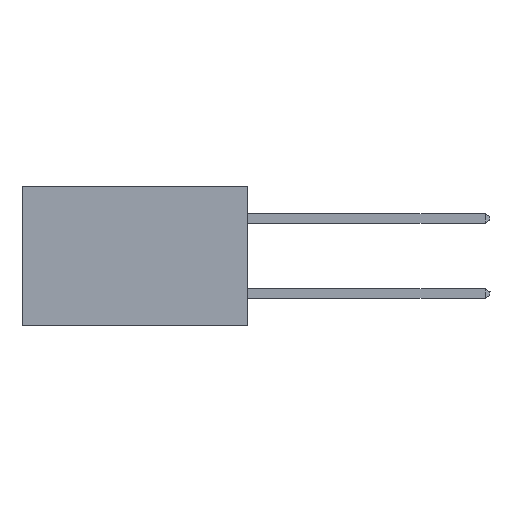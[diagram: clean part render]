
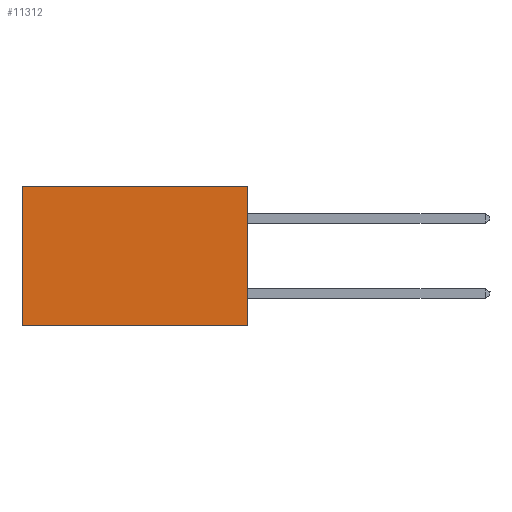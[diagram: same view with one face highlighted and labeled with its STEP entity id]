
A CAD part, left-side view. The second image highlights one B-rep face of the part: STEP entity #11312.
In plain terms, the highlighted planar face has unit normal (-1, 0, 0).
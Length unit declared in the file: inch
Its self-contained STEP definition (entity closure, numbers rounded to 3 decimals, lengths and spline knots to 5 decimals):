
#49 = EDGE_CURVE ( 'NONE', #9628, #14925, #16740, .T. ) ;
#114 = ORIENTED_EDGE ( 'NONE', *, *, #18227, .T. ) ;
#130 = CARTESIAN_POINT ( 'NONE',  ( 0.298, 0., -0.37 ) ) ;
#2113 = VECTOR ( 'NONE', #4062, 39.37008 ) ;
#2591 = VERTEX_POINT ( 'NONE', #6976 ) ;
#2922 = PLANE ( 'NONE',  #6608 ) ;
#3914 = ORIENTED_EDGE ( 'NONE', *, *, #7515, .T. ) ;
#4062 = DIRECTION ( 'NONE',  ( 0., 1., 0. ) ) ;
#4610 = DIRECTION ( 'NONE',  ( 0., 0., -1. ) ) ;
#4699 = DIRECTION ( 'NONE',  ( 1., 0., 0. ) ) ;
#5742 = VECTOR ( 'NONE', #8320, 39.37008 ) ;
#5875 = LINE ( 'NONE', #130, #2113 ) ;
#6608 = AXIS2_PLACEMENT_3D ( 'NONE', #10357, #4699, #21633 ) ;
#6976 = CARTESIAN_POINT ( 'NONE',  ( 0.298, 0.6, 0. ) ) ;
#7101 = CARTESIAN_POINT ( 'NONE',  ( 0.298, 0., 0. ) ) ;
#7515 = EDGE_CURVE ( 'NONE', #2591, #17797, #10724, .T. ) ;
#8263 = CARTESIAN_POINT ( 'NONE',  ( 0.298, 0.6, -0.37 ) ) ;
#8320 = DIRECTION ( 'NONE',  ( 0., 0., -1. ) ) ;
#9628 = VERTEX_POINT ( 'NONE', #7101 ) ;
#9670 = ORIENTED_EDGE ( 'NONE', *, *, #49, .F. ) ;
#10357 = CARTESIAN_POINT ( 'NONE',  ( 0.298, 0., 0. ) ) ;
#10724 = LINE ( 'NONE', #19567, #5742 ) ;
#11312 = ADVANCED_FACE ( 'NONE', ( #20436 ), #2922, .F. ) ;
#11809 = VECTOR ( 'NONE', #4610, 39.37008 ) ;
#12105 = EDGE_CURVE ( 'NONE', #14925, #17797, #5875, .T. ) ;
#13622 = VECTOR ( 'NONE', #18709, 39.37008 ) ;
#14925 = VERTEX_POINT ( 'NONE', #23064 ) ;
#14986 = EDGE_LOOP ( 'NONE', ( #3914, #18540, #9670, #114 ) ) ;
#16740 = LINE ( 'NONE', #19393, #11809 ) ;
#16852 = CARTESIAN_POINT ( 'NONE',  ( 0.298, 0., 0. ) ) ;
#17797 = VERTEX_POINT ( 'NONE', #8263 ) ;
#18227 = EDGE_CURVE ( 'NONE', #9628, #2591, #23164, .T. ) ;
#18540 = ORIENTED_EDGE ( 'NONE', *, *, #12105, .F. ) ;
#18709 = DIRECTION ( 'NONE',  ( 0., 1., 0. ) ) ;
#19393 = CARTESIAN_POINT ( 'NONE',  ( 0.298, 0., 0. ) ) ;
#19567 = CARTESIAN_POINT ( 'NONE',  ( 0.298, 0.6, 0. ) ) ;
#20436 = FACE_OUTER_BOUND ( 'NONE', #14986, .T. ) ;
#21633 = DIRECTION ( 'NONE',  ( 0., 0., -1. ) ) ;
#23064 = CARTESIAN_POINT ( 'NONE',  ( 0.298, 0., -0.37 ) ) ;
#23164 = LINE ( 'NONE', #16852, #13622 ) ;
